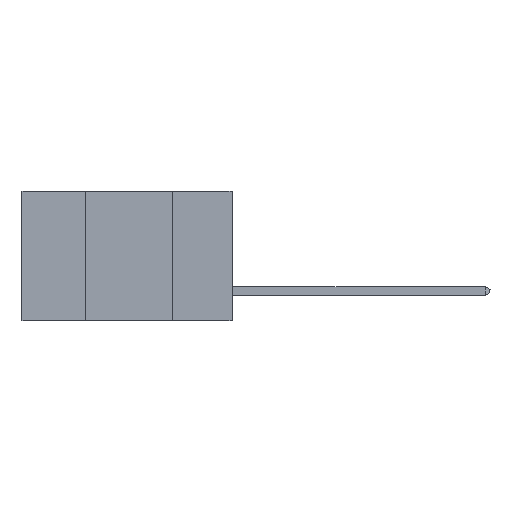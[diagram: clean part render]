
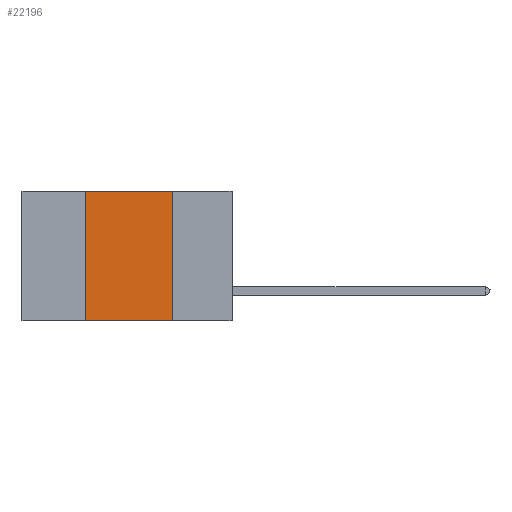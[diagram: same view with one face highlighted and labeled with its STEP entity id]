
A CAD part, left-side view. The second image highlights one B-rep face of the part: STEP entity #22196.
In plain terms, the highlighted planar face has unit normal (-1, 0, 0).
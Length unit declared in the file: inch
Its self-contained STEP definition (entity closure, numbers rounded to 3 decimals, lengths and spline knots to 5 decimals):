
#285 = DIRECTION ( 'NONE',  ( 0., -1., 0. ) ) ;
#713 = CARTESIAN_POINT ( 'NONE',  ( 0., 0.42, -0.37 ) ) ;
#967 = FACE_OUTER_BOUND ( 'NONE', #8772, .T. ) ;
#1081 = ORIENTED_EDGE ( 'NONE', *, *, #9453, .F. ) ;
#3234 = PLANE ( 'NONE',  #10488 ) ;
#5092 = VECTOR ( 'NONE', #18206, 39.37008 ) ;
#5863 = EDGE_CURVE ( 'NONE', #14719, #22179, #19067, .T. ) ;
#6226 = CARTESIAN_POINT ( 'NONE',  ( 0., 0.42, 0. ) ) ;
#6669 = DIRECTION ( 'NONE',  ( 0., 0., -1. ) ) ;
#6748 = LINE ( 'NONE', #9574, #12870 ) ;
#7258 = CARTESIAN_POINT ( 'NONE',  ( 0., 0.6, 0. ) ) ;
#7803 = VERTEX_POINT ( 'NONE', #18572 ) ;
#8772 = EDGE_LOOP ( 'NONE', ( #1081, #17034, #21254, #15535 ) ) ;
#9453 = EDGE_CURVE ( 'NONE', #7803, #22179, #6748, .T. ) ;
#9574 = CARTESIAN_POINT ( 'NONE',  ( 0., 0.17, 0. ) ) ;
#9794 = CARTESIAN_POINT ( 'NONE',  ( 0., 0.17, -0.37 ) ) ;
#10488 = AXIS2_PLACEMENT_3D ( 'NONE', #15207, #16919, #6669 ) ;
#10779 = EDGE_CURVE ( 'NONE', #14719, #16430, #21427, .T. ) ;
#12870 = VECTOR ( 'NONE', #16493, 39.37008 ) ;
#14719 = VERTEX_POINT ( 'NONE', #713 ) ;
#14871 = EDGE_CURVE ( 'NONE', #16430, #7803, #19244, .T. ) ;
#15207 = CARTESIAN_POINT ( 'NONE',  ( 0., 0.6, 0. ) ) ;
#15535 = ORIENTED_EDGE ( 'NONE', *, *, #5863, .T. ) ;
#15621 = CARTESIAN_POINT ( 'NONE',  ( 0., 0.6, -0.37 ) ) ;
#16430 = VERTEX_POINT ( 'NONE', #20632 ) ;
#16493 = DIRECTION ( 'NONE',  ( 0., 0., -1. ) ) ;
#16542 = VECTOR ( 'NONE', #285, 39.37008 ) ;
#16919 = DIRECTION ( 'NONE',  ( 1., 0., 0. ) ) ;
#17034 = ORIENTED_EDGE ( 'NONE', *, *, #14871, .F. ) ;
#18206 = DIRECTION ( 'NONE',  ( 0., 0., 1. ) ) ;
#18572 = CARTESIAN_POINT ( 'NONE',  ( 0., 0.17, 0. ) ) ;
#19067 = LINE ( 'NONE', #15621, #19588 ) ;
#19244 = LINE ( 'NONE', #7258, #16542 ) ;
#19588 = VECTOR ( 'NONE', #21084, 39.37008 ) ;
#20632 = CARTESIAN_POINT ( 'NONE',  ( 0., 0.42, 0. ) ) ;
#21084 = DIRECTION ( 'NONE',  ( 0., -1., 0. ) ) ;
#21254 = ORIENTED_EDGE ( 'NONE', *, *, #10779, .F. ) ;
#21427 = LINE ( 'NONE', #6226, #5092 ) ;
#22179 = VERTEX_POINT ( 'NONE', #9794 ) ;
#22196 = ADVANCED_FACE ( 'NONE', ( #967 ), #3234, .F. ) ;
